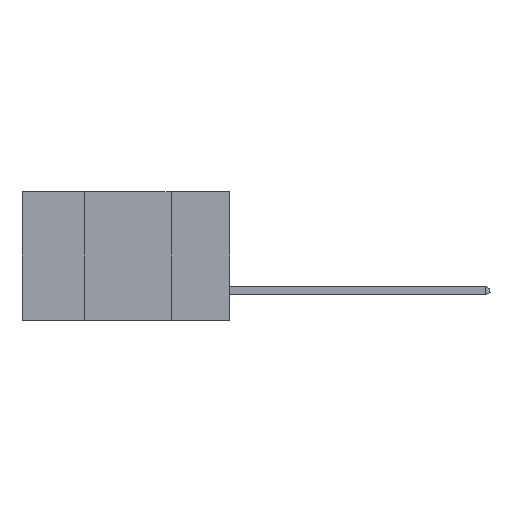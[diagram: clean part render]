
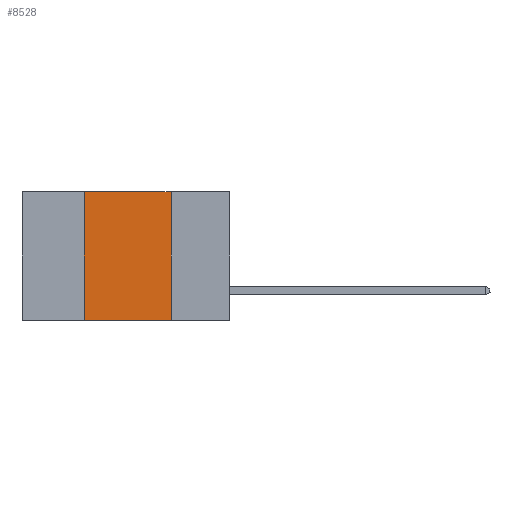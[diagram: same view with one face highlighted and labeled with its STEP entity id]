
A CAD part, left-side view. The second image highlights one B-rep face of the part: STEP entity #8528.
In plain terms, the highlighted planar face has unit normal (-1, 0, 0).
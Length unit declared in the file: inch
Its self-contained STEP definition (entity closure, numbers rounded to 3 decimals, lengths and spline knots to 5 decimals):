
#767 = VERTEX_POINT ( 'NONE', #2613 ) ;
#1135 = DIRECTION ( 'NONE',  ( 0., 0., 1. ) ) ;
#1902 = VECTOR ( 'NONE', #12551, 39.37008 ) ;
#1912 = ORIENTED_EDGE ( 'NONE', *, *, #20279, .F. ) ;
#2613 = CARTESIAN_POINT ( 'NONE',  ( 0., 0.42, 0. ) ) ;
#3659 = LINE ( 'NONE', #6808, #19881 ) ;
#3984 = DIRECTION ( 'NONE',  ( 0., 0., -1. ) ) ;
#4142 = CARTESIAN_POINT ( 'NONE',  ( 0., 0.17, 0. ) ) ;
#4608 = EDGE_LOOP ( 'NONE', ( #6809, #1912, #14739, #18512 ) ) ;
#5346 = VERTEX_POINT ( 'NONE', #4142 ) ;
#5473 = VERTEX_POINT ( 'NONE', #12903 ) ;
#6808 = CARTESIAN_POINT ( 'NONE',  ( 0., 0.6, -0.37 ) ) ;
#6809 = ORIENTED_EDGE ( 'NONE', *, *, #14960, .F. ) ;
#7537 = EDGE_CURVE ( 'NONE', #5473, #12649, #3659, .T. ) ;
#8528 = ADVANCED_FACE ( 'NONE', ( #17344 ), #12060, .F. ) ;
#8621 = DIRECTION ( 'NONE',  ( 1., 0., 0. ) ) ;
#9658 = EDGE_CURVE ( 'NONE', #5473, #767, #12580, .T. ) ;
#10995 = DIRECTION ( 'NONE',  ( 0., 0., -1. ) ) ;
#11192 = CARTESIAN_POINT ( 'NONE',  ( 0., 0.6, 0. ) ) ;
#12060 = PLANE ( 'NONE',  #12876 ) ;
#12390 = LINE ( 'NONE', #11192, #1902 ) ;
#12551 = DIRECTION ( 'NONE',  ( 0., -1., 0. ) ) ;
#12580 = LINE ( 'NONE', #19794, #13575 ) ;
#12649 = VERTEX_POINT ( 'NONE', #18969 ) ;
#12876 = AXIS2_PLACEMENT_3D ( 'NONE', #13380, #8621, #3984 ) ;
#12903 = CARTESIAN_POINT ( 'NONE',  ( 0., 0.42, -0.37 ) ) ;
#13380 = CARTESIAN_POINT ( 'NONE',  ( 0., 0.6, 0. ) ) ;
#13575 = VECTOR ( 'NONE', #1135, 39.37008 ) ;
#13944 = DIRECTION ( 'NONE',  ( 0., -1., 0. ) ) ;
#14212 = CARTESIAN_POINT ( 'NONE',  ( 0., 0.17, 0. ) ) ;
#14739 = ORIENTED_EDGE ( 'NONE', *, *, #9658, .F. ) ;
#14960 = EDGE_CURVE ( 'NONE', #5346, #12649, #17291, .T. ) ;
#16799 = VECTOR ( 'NONE', #10995, 39.37008 ) ;
#17291 = LINE ( 'NONE', #14212, #16799 ) ;
#17344 = FACE_OUTER_BOUND ( 'NONE', #4608, .T. ) ;
#18512 = ORIENTED_EDGE ( 'NONE', *, *, #7537, .T. ) ;
#18969 = CARTESIAN_POINT ( 'NONE',  ( 0., 0.17, -0.37 ) ) ;
#19794 = CARTESIAN_POINT ( 'NONE',  ( 0., 0.42, 0. ) ) ;
#19881 = VECTOR ( 'NONE', #13944, 39.37008 ) ;
#20279 = EDGE_CURVE ( 'NONE', #767, #5346, #12390, .T. ) ;
